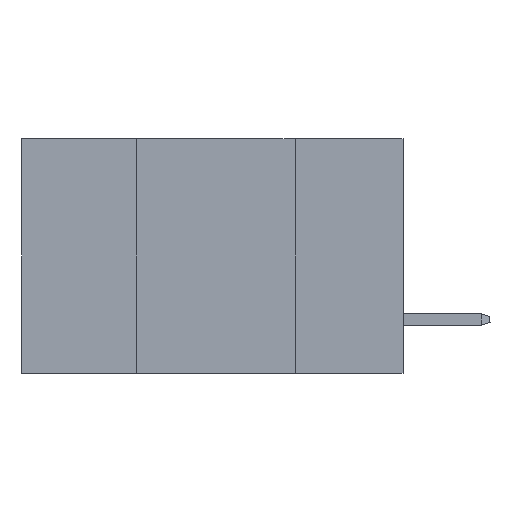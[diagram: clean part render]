
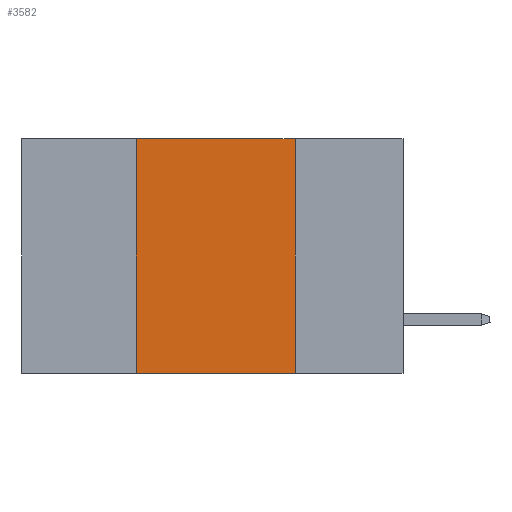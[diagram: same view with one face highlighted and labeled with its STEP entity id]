
A CAD part, left-side view. The second image highlights one B-rep face of the part: STEP entity #3582.
In plain terms, the highlighted planar face has unit normal (-1, 0, 0).
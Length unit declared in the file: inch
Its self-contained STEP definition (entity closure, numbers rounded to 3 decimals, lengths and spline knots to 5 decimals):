
#428 = VECTOR ( 'NONE', #4238, 39.37008 ) ;
#1604 = DIRECTION ( 'NONE',  ( 0., -1., 0. ) ) ;
#3565 = VERTEX_POINT ( 'NONE', #27960 ) ;
#3582 = ADVANCED_FACE ( 'NONE', ( #15318 ), #10908, .F. ) ;
#3871 = VECTOR ( 'NONE', #27676, 39.37008 ) ;
#4238 = DIRECTION ( 'NONE',  ( 0., 0., -1. ) ) ;
#5936 = ORIENTED_EDGE ( 'NONE', *, *, #20691, .F. ) ;
#6024 = VECTOR ( 'NONE', #1604, 39.37008 ) ;
#6679 = VECTOR ( 'NONE', #15586, 39.37008 ) ;
#6784 = DIRECTION ( 'NONE',  ( 1., 0., 0. ) ) ;
#6905 = ORIENTED_EDGE ( 'NONE', *, *, #25678, .F. ) ;
#6922 = VERTEX_POINT ( 'NONE', #26938 ) ;
#7935 = EDGE_LOOP ( 'NONE', ( #6905, #5936, #16277, #15735 ) ) ;
#10177 = LINE ( 'NONE', #23124, #6024 ) ;
#10908 = PLANE ( 'NONE',  #18465 ) ;
#12638 = CARTESIAN_POINT ( 'NONE',  ( 0., 0.6, 0. ) ) ;
#13529 = EDGE_CURVE ( 'NONE', #3565, #18018, #10177, .T. ) ;
#14785 = VERTEX_POINT ( 'NONE', #21651 ) ;
#15197 = LINE ( 'NONE', #23736, #428 ) ;
#15318 = FACE_OUTER_BOUND ( 'NONE', #7935, .T. ) ;
#15586 = DIRECTION ( 'NONE',  ( 0., -1., 0. ) ) ;
#15735 = ORIENTED_EDGE ( 'NONE', *, *, #13529, .T. ) ;
#16277 = ORIENTED_EDGE ( 'NONE', *, *, #16964, .F. ) ;
#16964 = EDGE_CURVE ( 'NONE', #3565, #14785, #19299, .T. ) ;
#18018 = VERTEX_POINT ( 'NONE', #23786 ) ;
#18465 = AXIS2_PLACEMENT_3D ( 'NONE', #12638, #6784, #19576 ) ;
#19299 = LINE ( 'NONE', #21455, #3871 ) ;
#19576 = DIRECTION ( 'NONE',  ( 0., 0., -1. ) ) ;
#20691 = EDGE_CURVE ( 'NONE', #14785, #6922, #24529, .T. ) ;
#21455 = CARTESIAN_POINT ( 'NONE',  ( 0., 0.42, 0. ) ) ;
#21651 = CARTESIAN_POINT ( 'NONE',  ( 0., 0.42, 0. ) ) ;
#23124 = CARTESIAN_POINT ( 'NONE',  ( 0., 0.6, -0.37 ) ) ;
#23736 = CARTESIAN_POINT ( 'NONE',  ( 0., 0.17, 0. ) ) ;
#23786 = CARTESIAN_POINT ( 'NONE',  ( 0., 0.17, -0.37 ) ) ;
#24529 = LINE ( 'NONE', #26511, #6679 ) ;
#25678 = EDGE_CURVE ( 'NONE', #6922, #18018, #15197, .T. ) ;
#26511 = CARTESIAN_POINT ( 'NONE',  ( 0., 0.6, 0. ) ) ;
#26938 = CARTESIAN_POINT ( 'NONE',  ( 0., 0.17, 0. ) ) ;
#27676 = DIRECTION ( 'NONE',  ( 0., 0., 1. ) ) ;
#27960 = CARTESIAN_POINT ( 'NONE',  ( 0., 0.42, -0.37 ) ) ;
